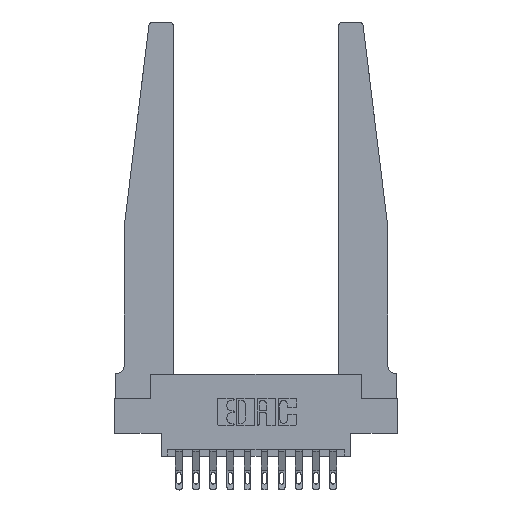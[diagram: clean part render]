
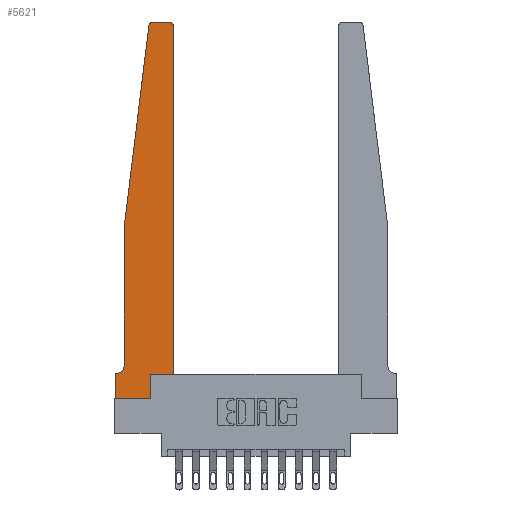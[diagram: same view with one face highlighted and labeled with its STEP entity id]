
A CAD part, top view. The second image highlights one B-rep face of the part: STEP entity #5621.
In plain terms, the highlighted planar face has unit normal (0, 0, 1).
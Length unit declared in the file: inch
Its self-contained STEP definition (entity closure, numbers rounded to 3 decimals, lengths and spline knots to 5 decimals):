
#298 = CARTESIAN_POINT ( 'NONE',  ( 0.065, 0.2375, 0.37 ) ) ;
#476 = EDGE_CURVE ( 'NONE', #12031, #4016, #7707, .T. ) ;
#496 = DIRECTION ( 'NONE',  ( 0., 1., 0. ) ) ;
#524 = CARTESIAN_POINT ( 'NONE',  ( 0., 0., 0.37 ) ) ;
#730 = CARTESIAN_POINT ( 'NONE',  ( 0., 0., 0.37 ) ) ;
#737 = VERTEX_POINT ( 'NONE', #10717 ) ;
#1107 = ORIENTED_EDGE ( 'NONE', *, *, #3332, .T. ) ;
#1108 = LINE ( 'NONE', #14852, #10622 ) ;
#1141 = CARTESIAN_POINT ( 'NONE',  ( 0.425, 0.18, 0.37 ) ) ;
#1151 = DIRECTION ( 'NONE',  ( 0., -1., 0. ) ) ;
#1213 = LINE ( 'NONE', #13390, #4510 ) ;
#1371 = CARTESIAN_POINT ( 'NONE',  ( 0.24675, 2.72367, 0.37 ) ) ;
#1676 = VERTEX_POINT ( 'NONE', #10984 ) ;
#1696 = DIRECTION ( 'NONE',  ( 0., 0., -1. ) ) ;
#1937 = PLANE ( 'NONE',  #15594 ) ;
#2142 = VERTEX_POINT ( 'NONE', #298 ) ;
#2230 = DIRECTION ( 'NONE',  ( 0., 0., 1. ) ) ;
#2879 = EDGE_CURVE ( 'NONE', #1676, #15011, #15007, .T. ) ;
#3067 = CARTESIAN_POINT ( 'NONE',  ( 0.27653, 2.72, 0.37 ) ) ;
#3185 = CARTESIAN_POINT ( 'NONE',  ( 0., 0.1875, 0.37 ) ) ;
#3332 = EDGE_CURVE ( 'NONE', #2142, #7999, #12453, .T. ) ;
#3469 = DIRECTION ( 'NONE',  ( -0.122, -0.992, 0. ) ) ;
#3642 = EDGE_CURVE ( 'NONE', #11284, #737, #1213, .T. ) ;
#3718 = EDGE_CURVE ( 'NONE', #737, #2142, #4123, .T. ) ;
#3735 = DIRECTION ( 'NONE',  ( -1., 0., 0. ) ) ;
#4016 = VERTEX_POINT ( 'NONE', #524 ) ;
#4123 = LINE ( 'NONE', #9823, #12832 ) ;
#4262 = CARTESIAN_POINT ( 'NONE',  ( 0.425, 0.18, 0.37 ) ) ;
#4324 = DIRECTION ( 'NONE',  ( 1., 0., 0. ) ) ;
#4431 = DIRECTION ( 'NONE',  ( 1., 0., 0. ) ) ;
#4510 = VECTOR ( 'NONE', #3469, 39.37008 ) ;
#4892 = VERTEX_POINT ( 'NONE', #14102 ) ;
#5034 = AXIS2_PLACEMENT_3D ( 'NONE', #9663, #2230, #10898 ) ;
#5121 = VECTOR ( 'NONE', #496, 39.37008 ) ;
#5543 = CARTESIAN_POINT ( 'NONE',  ( 0., 0.1875, 0.37 ) ) ;
#5621 = ADVANCED_FACE ( 'NONE', ( #11132 ), #1937, .T. ) ;
#5989 = EDGE_LOOP ( 'NONE', ( #6927, #10222, #10620, #15471, #1107, #14691, #8110, #15082, #11774, #12153, #13323, #7913 ) ) ;
#6114 = VECTOR ( 'NONE', #6967, 39.37008 ) ;
#6927 = ORIENTED_EDGE ( 'NONE', *, *, #14406, .T. ) ;
#6967 = DIRECTION ( 'NONE',  ( 1., 0., 0. ) ) ;
#7095 = DIRECTION ( 'NONE',  ( -1., 0., 0. ) ) ;
#7206 = VERTEX_POINT ( 'NONE', #11106 ) ;
#7319 = VECTOR ( 'NONE', #12126, 39.37008 ) ;
#7362 = CIRCLE ( 'NONE', #5034, 0.03 ) ;
#7707 = LINE ( 'NONE', #14642, #7319 ) ;
#7913 = ORIENTED_EDGE ( 'NONE', *, *, #8706, .T. ) ;
#7999 = VERTEX_POINT ( 'NONE', #14277 ) ;
#8073 = VECTOR ( 'NONE', #7095, 39.37008 ) ;
#8110 = ORIENTED_EDGE ( 'NONE', *, *, #476, .T. ) ;
#8112 = VECTOR ( 'NONE', #14646, 39.37008 ) ;
#8554 = CIRCLE ( 'NONE', #15200, 0.03 ) ;
#8688 = DIRECTION ( 'NONE',  ( 0., 1., 0. ) ) ;
#8693 = CARTESIAN_POINT ( 'NONE',  ( 0.25, 2.75, 0.37 ) ) ;
#8706 = EDGE_CURVE ( 'NONE', #15011, #12414, #7362, .T. ) ;
#9140 = CARTESIAN_POINT ( 'NONE',  ( 0.015, 0.2375, 0.37 ) ) ;
#9406 = LINE ( 'NONE', #730, #6114 ) ;
#9663 = CARTESIAN_POINT ( 'NONE',  ( 0.395, 2.72, 0.37 ) ) ;
#9823 = CARTESIAN_POINT ( 'NONE',  ( 0.065, 1.25, 0.37 ) ) ;
#10086 = EDGE_CURVE ( 'NONE', #7206, #1676, #11391, .T. ) ;
#10140 = EDGE_CURVE ( 'NONE', #13222, #7206, #1108, .T. ) ;
#10222 = ORIENTED_EDGE ( 'NONE', *, *, #16080, .T. ) ;
#10371 = DIRECTION ( 'NONE',  ( -1., 0., 0. ) ) ;
#10620 = ORIENTED_EDGE ( 'NONE', *, *, #3642, .T. ) ;
#10622 = VECTOR ( 'NONE', #8688, 39.37008 ) ;
#10717 = CARTESIAN_POINT ( 'NONE',  ( 0.065, 1.25, 0.37 ) ) ;
#10898 = DIRECTION ( 'NONE',  ( 1., 0., 0. ) ) ;
#10984 = CARTESIAN_POINT ( 'NONE',  ( 0.425, 0.18, 0.37 ) ) ;
#11106 = CARTESIAN_POINT ( 'NONE',  ( 0.2605, 0.18, 0.37 ) ) ;
#11132 = FACE_OUTER_BOUND ( 'NONE', #5989, .T. ) ;
#11284 = VERTEX_POINT ( 'NONE', #1371 ) ;
#11391 = LINE ( 'NONE', #1141, #8112 ) ;
#11700 = LINE ( 'NONE', #8693, #14615 ) ;
#11739 = DIRECTION ( 'NONE',  ( 0., 0., 1. ) ) ;
#11774 = ORIENTED_EDGE ( 'NONE', *, *, #10140, .T. ) ;
#11850 = DIRECTION ( 'NONE',  ( 0., 0., 1. ) ) ;
#12031 = VERTEX_POINT ( 'NONE', #5543 ) ;
#12126 = DIRECTION ( 'NONE',  ( 0., -1., 0. ) ) ;
#12153 = ORIENTED_EDGE ( 'NONE', *, *, #10086, .T. ) ;
#12378 = CARTESIAN_POINT ( 'NONE',  ( 0.395, 2.75, 0.37 ) ) ;
#12414 = VERTEX_POINT ( 'NONE', #12378 ) ;
#12453 = CIRCLE ( 'NONE', #14218, 0.05 ) ;
#12832 = VECTOR ( 'NONE', #1151, 39.37008 ) ;
#12977 = EDGE_CURVE ( 'NONE', #7999, #12031, #14265, .T. ) ;
#13222 = VERTEX_POINT ( 'NONE', #14894 ) ;
#13261 = CARTESIAN_POINT ( 'NONE',  ( 0.065, 0.1875, 0.37 ) ) ;
#13323 = ORIENTED_EDGE ( 'NONE', *, *, #2879, .T. ) ;
#13390 = CARTESIAN_POINT ( 'NONE',  ( 0.065, 1.25, 0.37 ) ) ;
#13594 = EDGE_CURVE ( 'NONE', #4016, #13222, #9406, .T. ) ;
#14102 = CARTESIAN_POINT ( 'NONE',  ( 0.27653, 2.75, 0.37 ) ) ;
#14218 = AXIS2_PLACEMENT_3D ( 'NONE', #9140, #1696, #10371 ) ;
#14265 = LINE ( 'NONE', #13261, #8073 ) ;
#14277 = CARTESIAN_POINT ( 'NONE',  ( 0.015, 0.1875, 0.37 ) ) ;
#14406 = EDGE_CURVE ( 'NONE', #12414, #4892, #11700, .T. ) ;
#14615 = VECTOR ( 'NONE', #3735, 39.37008 ) ;
#14642 = CARTESIAN_POINT ( 'NONE',  ( 0., 0., 0.37 ) ) ;
#14646 = DIRECTION ( 'NONE',  ( 1., 0., 0. ) ) ;
#14691 = ORIENTED_EDGE ( 'NONE', *, *, #12977, .T. ) ;
#14852 = CARTESIAN_POINT ( 'NONE',  ( 0.2605, 0.18, 0.37 ) ) ;
#14894 = CARTESIAN_POINT ( 'NONE',  ( 0.2605, 0., 0.37 ) ) ;
#14900 = CARTESIAN_POINT ( 'NONE',  ( 0.425, 2.72, 0.37 ) ) ;
#15007 = LINE ( 'NONE', #4262, #5121 ) ;
#15011 = VERTEX_POINT ( 'NONE', #14900 ) ;
#15082 = ORIENTED_EDGE ( 'NONE', *, *, #13594, .T. ) ;
#15200 = AXIS2_PLACEMENT_3D ( 'NONE', #3067, #11739, #4324 ) ;
#15471 = ORIENTED_EDGE ( 'NONE', *, *, #3718, .T. ) ;
#15594 = AXIS2_PLACEMENT_3D ( 'NONE', #3185, #11850, #4431 ) ;
#16080 = EDGE_CURVE ( 'NONE', #4892, #11284, #8554, .T. ) ;
